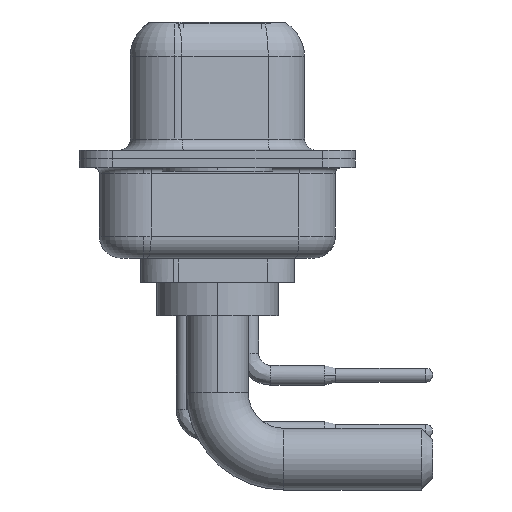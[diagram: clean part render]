
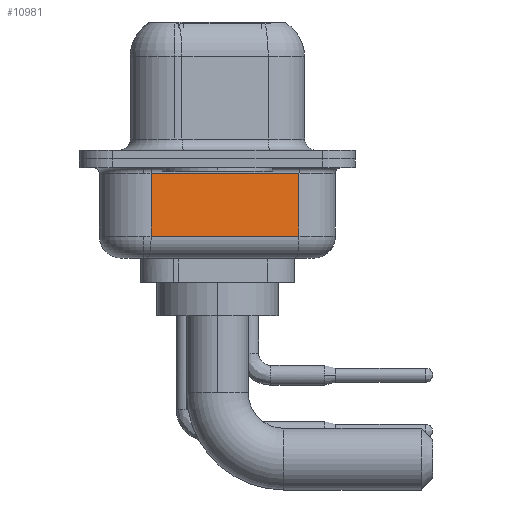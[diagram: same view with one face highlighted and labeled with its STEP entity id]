
A CAD part, left-side view. The second image highlights one B-rep face of the part: STEP entity #10981.
In plain terms, the highlighted planar face has unit normal (-0.985, -0.174, 0).
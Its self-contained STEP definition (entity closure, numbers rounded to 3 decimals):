
#366 = LINE ( 'NONE', #12627, #2823 ) ;
#678 = ORIENTED_EDGE ( 'NONE', *, *, #9915, .F. ) ;
#917 = AXIS2_PLACEMENT_3D ( 'NONE', #20762, #9967, #22617 ) ;
#1653 = DIRECTION ( 'NONE',  ( 0., 0., 1. ) ) ;
#2823 = VECTOR ( 'NONE', #5283, 1000. ) ;
#2853 = ORIENTED_EDGE ( 'NONE', *, *, #18082, .T. ) ;
#4522 = VERTEX_POINT ( 'NONE', #8440 ) ;
#4824 = FACE_OUTER_BOUND ( 'NONE', #7408, .T. ) ;
#4825 = CARTESIAN_POINT ( 'NONE',  ( 4.062, -3.697, -0.65 ) ) ;
#5283 = DIRECTION ( 'NONE',  ( 0.174, -0.985, 0. ) ) ;
#5300 = VERTEX_POINT ( 'NONE', #13054 ) ;
#5700 = ORIENTED_EDGE ( 'NONE', *, *, #21980, .T. ) ;
#6369 = CARTESIAN_POINT ( 'NONE',  ( 4.062, -3.697, -3.5 ) ) ;
#7408 = EDGE_LOOP ( 'NONE', ( #678, #2853, #5700, #18287 ) ) ;
#8440 = CARTESIAN_POINT ( 'NONE',  ( 2.88, 3.003, -0.65 ) ) ;
#8445 = PLANE ( 'NONE',  #917 ) ;
#8666 = CARTESIAN_POINT ( 'NONE',  ( 2.88, 3.003, -4.5 ) ) ;
#9795 = VECTOR ( 'NONE', #22498, 1000. ) ;
#9915 = EDGE_CURVE ( 'NONE', #5300, #4522, #20874, .T. ) ;
#9967 = DIRECTION ( 'NONE',  ( 0.985, 0.174, 0. ) ) ;
#10981 = ADVANCED_FACE ( 'NONE', ( #4824 ), #8445, .F. ) ;
#11114 = VECTOR ( 'NONE', #11793, 1000. ) ;
#11793 = DIRECTION ( 'NONE',  ( 0., 0., 1. ) ) ;
#11905 = LINE ( 'NONE', #20640, #11114 ) ;
#12238 = VERTEX_POINT ( 'NONE', #6369 ) ;
#12627 = CARTESIAN_POINT ( 'NONE',  ( 2.88, 3.003, -3.5 ) ) ;
#13054 = CARTESIAN_POINT ( 'NONE',  ( 2.88, 3.003, -3.5 ) ) ;
#15086 = CARTESIAN_POINT ( 'NONE',  ( 2.88, 3.003, -0.65 ) ) ;
#15732 = EDGE_CURVE ( 'NONE', #21600, #4522, #18236, .T. ) ;
#18082 = EDGE_CURVE ( 'NONE', #5300, #12238, #366, .T. ) ;
#18236 = LINE ( 'NONE', #15086, #9795 ) ;
#18287 = ORIENTED_EDGE ( 'NONE', *, *, #15732, .T. ) ;
#20571 = VECTOR ( 'NONE', #1653, 1000. ) ;
#20640 = CARTESIAN_POINT ( 'NONE',  ( 4.062, -3.697, -4.5 ) ) ;
#20762 = CARTESIAN_POINT ( 'NONE',  ( 2.88, 3.003, -4.5 ) ) ;
#20874 = LINE ( 'NONE', #8666, #20571 ) ;
#21600 = VERTEX_POINT ( 'NONE', #4825 ) ;
#21980 = EDGE_CURVE ( 'NONE', #12238, #21600, #11905, .T. ) ;
#22498 = DIRECTION ( 'NONE',  ( -0.174, 0.985, 0. ) ) ;
#22617 = DIRECTION ( 'NONE',  ( -0.174, 0.985, 0. ) ) ;
